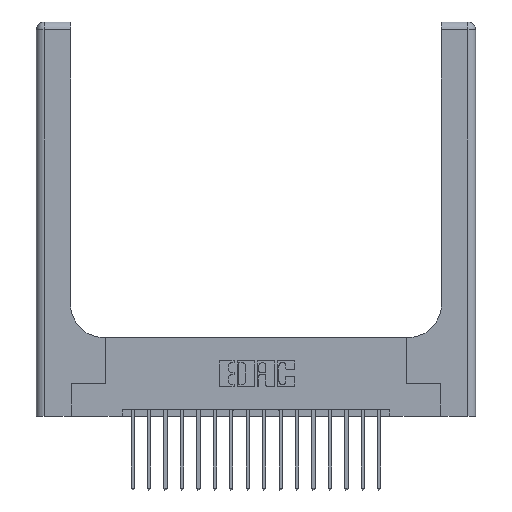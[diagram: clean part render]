
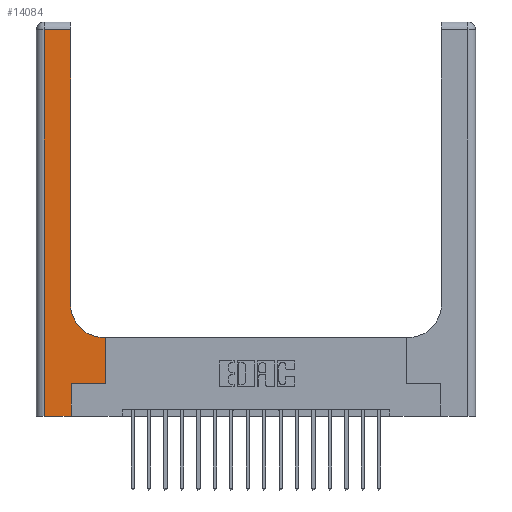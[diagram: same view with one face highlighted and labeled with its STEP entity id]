
A CAD part, top view. The second image highlights one B-rep face of the part: STEP entity #14084.
In plain terms, the highlighted planar face has unit normal (0, 0, 1).
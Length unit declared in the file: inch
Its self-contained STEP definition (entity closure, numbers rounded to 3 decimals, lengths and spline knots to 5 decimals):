
#69 = VERTEX_POINT ( 'NONE', #18548 ) ;
#272 = VERTEX_POINT ( 'NONE', #4371 ) ;
#590 = CARTESIAN_POINT ( 'NONE',  ( 0.26, 0.85, 0.37 ) ) ;
#624 = CARTESIAN_POINT ( 'NONE',  ( 0., 3., 0.37 ) ) ;
#936 = VECTOR ( 'NONE', #10592, 39.37008 ) ;
#991 = VERTEX_POINT ( 'NONE', #1602 ) ;
#1433 = ORIENTED_EDGE ( 'NONE', *, *, #12849, .T. ) ;
#1602 = CARTESIAN_POINT ( 'NONE',  ( 0.265, 0., 0.37 ) ) ;
#2489 = VERTEX_POINT ( 'NONE', #17789 ) ;
#2794 = VECTOR ( 'NONE', #7542, 39.37008 ) ;
#3027 = CARTESIAN_POINT ( 'NONE',  ( 0.51, 0.6, 0.37 ) ) ;
#3085 = VERTEX_POINT ( 'NONE', #16668 ) ;
#3290 = EDGE_CURVE ( 'NONE', #2489, #991, #5285, .T. ) ;
#3348 = CARTESIAN_POINT ( 'NONE',  ( 0.06, 3., 0.37 ) ) ;
#3654 = DIRECTION ( 'NONE',  ( 0., 1., 0. ) ) ;
#3800 = DIRECTION ( 'NONE',  ( -1., 0., 0. ) ) ;
#3957 = DIRECTION ( 'NONE',  ( -1., 0., 0. ) ) ;
#4371 = CARTESIAN_POINT ( 'NONE',  ( 0.26, 2.94, 0.37 ) ) ;
#4404 = EDGE_LOOP ( 'NONE', ( #5804, #4653, #15254, #8807, #10983, #9934, #6139, #6305, #1433 ) ) ;
#4536 = EDGE_CURVE ( 'NONE', #69, #3085, #14197, .T. ) ;
#4653 = ORIENTED_EDGE ( 'NONE', *, *, #9641, .T. ) ;
#4736 = LINE ( 'NONE', #10793, #2794 ) ;
#4885 = EDGE_CURVE ( 'NONE', #991, #8855, #12699, .T. ) ;
#4967 = VERTEX_POINT ( 'NONE', #590 ) ;
#5280 = EDGE_CURVE ( 'NONE', #4967, #272, #4736, .T. ) ;
#5285 = LINE ( 'NONE', #14193, #11556 ) ;
#5683 = CARTESIAN_POINT ( 'NONE',  ( 0., 2.94, 0.37 ) ) ;
#5747 = EDGE_CURVE ( 'NONE', #3085, #13675, #11022, .T. ) ;
#5804 = ORIENTED_EDGE ( 'NONE', *, *, #5280, .T. ) ;
#5960 = EDGE_CURVE ( 'NONE', #8855, #69, #6232, .T. ) ;
#6139 = ORIENTED_EDGE ( 'NONE', *, *, #4536, .T. ) ;
#6232 = LINE ( 'NONE', #15143, #936 ) ;
#6305 = ORIENTED_EDGE ( 'NONE', *, *, #5747, .T. ) ;
#6444 = DIRECTION ( 'NONE',  ( 0., -1., 0. ) ) ;
#6582 = DIRECTION ( 'NONE',  ( 0., 1., 0. ) ) ;
#6684 = DIRECTION ( 'NONE',  ( 0., 0., -1. ) ) ;
#6764 = DIRECTION ( 'NONE',  ( 1., 0., 0. ) ) ;
#7356 = CARTESIAN_POINT ( 'NONE',  ( 0.51, 0.85, 0.37 ) ) ;
#7542 = DIRECTION ( 'NONE',  ( 0., 1., 0. ) ) ;
#7668 = AXIS2_PLACEMENT_3D ( 'NONE', #624, #6684, #3800 ) ;
#8263 = FACE_OUTER_BOUND ( 'NONE', #4404, .T. ) ;
#8616 = CARTESIAN_POINT ( 'NONE',  ( 0.26, 0.6, 0.37 ) ) ;
#8807 = ORIENTED_EDGE ( 'NONE', *, *, #3290, .T. ) ;
#8855 = VERTEX_POINT ( 'NONE', #17127 ) ;
#9229 = VECTOR ( 'NONE', #6582, 39.37008 ) ;
#9243 = VECTOR ( 'NONE', #3654, 39.37008 ) ;
#9641 = EDGE_CURVE ( 'NONE', #272, #10658, #14794, .T. ) ;
#9934 = ORIENTED_EDGE ( 'NONE', *, *, #5960, .T. ) ;
#10108 = CARTESIAN_POINT ( 'NONE',  ( 0.06, 2.94, 0.37 ) ) ;
#10152 = DIRECTION ( 'NONE',  ( -1., 0., 0. ) ) ;
#10219 = VECTOR ( 'NONE', #10152, 39.37008 ) ;
#10592 = DIRECTION ( 'NONE',  ( 1., 0., 0. ) ) ;
#10658 = VERTEX_POINT ( 'NONE', #10108 ) ;
#10744 = VECTOR ( 'NONE', #3957, 39.37008 ) ;
#10793 = CARTESIAN_POINT ( 'NONE',  ( 0.26, 3., 0.37 ) ) ;
#10983 = ORIENTED_EDGE ( 'NONE', *, *, #4885, .T. ) ;
#11022 = LINE ( 'NONE', #8616, #10744 ) ;
#11137 = CARTESIAN_POINT ( 'NONE',  ( 0.528, 0.25, 0.37 ) ) ;
#11556 = VECTOR ( 'NONE', #6764, 39.37008 ) ;
#12699 = LINE ( 'NONE', #17038, #9243 ) ;
#12849 = EDGE_CURVE ( 'NONE', #13675, #4967, #18004, .T. ) ;
#13675 = VERTEX_POINT ( 'NONE', #3027 ) ;
#14084 = ADVANCED_FACE ( 'NONE', ( #8263 ), #17264, .F. ) ;
#14193 = CARTESIAN_POINT ( 'NONE',  ( 0., 0., 0.37 ) ) ;
#14197 = LINE ( 'NONE', #11137, #9229 ) ;
#14794 = LINE ( 'NONE', #5683, #10219 ) ;
#14995 = DIRECTION ( 'NONE',  ( 1., 0., 0. ) ) ;
#15143 = CARTESIAN_POINT ( 'NONE',  ( 0.265, 0.25, 0.37 ) ) ;
#15254 = ORIENTED_EDGE ( 'NONE', *, *, #19556, .T. ) ;
#15807 = AXIS2_PLACEMENT_3D ( 'NONE', #7356, #17855, #14995 ) ;
#16668 = CARTESIAN_POINT ( 'NONE',  ( 0.528, 0.6, 0.37 ) ) ;
#16817 = LINE ( 'NONE', #3348, #18852 ) ;
#17038 = CARTESIAN_POINT ( 'NONE',  ( 0.265, 0., 0.37 ) ) ;
#17127 = CARTESIAN_POINT ( 'NONE',  ( 0.265, 0.25, 0.37 ) ) ;
#17264 = PLANE ( 'NONE',  #7668 ) ;
#17789 = CARTESIAN_POINT ( 'NONE',  ( 0.06, 0., 0.37 ) ) ;
#17855 = DIRECTION ( 'NONE',  ( 0., 0., -1. ) ) ;
#18004 = CIRCLE ( 'NONE', #15807, 0.25 ) ;
#18548 = CARTESIAN_POINT ( 'NONE',  ( 0.528, 0.25, 0.37 ) ) ;
#18852 = VECTOR ( 'NONE', #6444, 39.37008 ) ;
#19556 = EDGE_CURVE ( 'NONE', #10658, #2489, #16817, .T. ) ;
